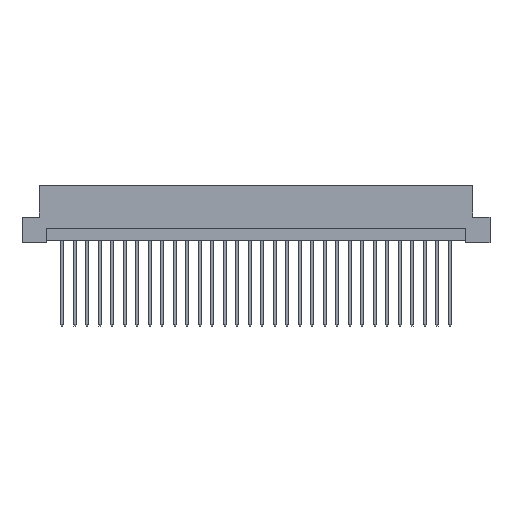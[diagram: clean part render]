
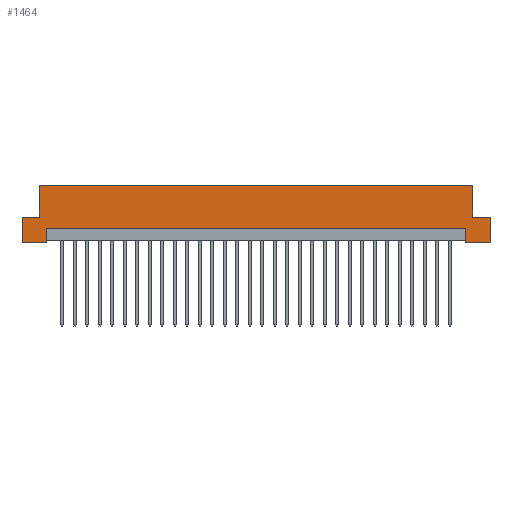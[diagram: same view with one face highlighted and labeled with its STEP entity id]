
A CAD part, front view. The second image highlights one B-rep face of the part: STEP entity #1464.
In plain terms, the highlighted planar face has unit normal (0, -1, 0).
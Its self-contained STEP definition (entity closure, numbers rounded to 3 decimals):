
#237 = EDGE_CURVE ( 'NONE', #8141, #10789, #5623, .T. ) ;
#249 = ORIENTED_EDGE ( 'NONE', *, *, #237, .F. ) ;
#251 = VECTOR ( 'NONE', #8295, 1000. ) ;
#266 = CARTESIAN_POINT ( 'NONE',  ( -44., 0., 5.2 ) ) ;
#455 = EDGE_CURVE ( 'NONE', #5462, #10347, #2420, .T. ) ;
#1003 = DIRECTION ( 'NONE',  ( 0., 0., -1. ) ) ;
#1464 = ADVANCED_FACE ( 'NONE', ( #6351 ), #17099, .F. ) ;
#1670 = VERTEX_POINT ( 'NONE', #11177 ) ;
#1821 = ORIENTED_EDGE ( 'NONE', *, *, #17286, .T. ) ;
#2420 = LINE ( 'NONE', #6477, #3957 ) ;
#2561 = EDGE_CURVE ( 'NONE', #5462, #15795, #7769, .T. ) ;
#2587 = VERTEX_POINT ( 'NONE', #3635 ) ;
#2605 = VECTOR ( 'NONE', #6681, 1000. ) ;
#2892 = CARTESIAN_POINT ( 'NONE',  ( -47.5, 0., 11.6 ) ) ;
#2977 = CARTESIAN_POINT ( 'NONE',  ( -47.5, 0., 5.2 ) ) ;
#3029 = CARTESIAN_POINT ( 'NONE',  ( -47.5, 0., 0. ) ) ;
#3141 = CARTESIAN_POINT ( 'NONE',  ( -47.5, 0., 0. ) ) ;
#3635 = CARTESIAN_POINT ( 'NONE',  ( 44., 0., 5.2 ) ) ;
#3672 = DIRECTION ( 'NONE',  ( 0., 0., -1. ) ) ;
#3743 = DIRECTION ( 'NONE',  ( -1., 0., 0. ) ) ;
#3848 = CARTESIAN_POINT ( 'NONE',  ( 44., 0., 5.2 ) ) ;
#3914 = VECTOR ( 'NONE', #5769, 1000. ) ;
#3940 = EDGE_CURVE ( 'NONE', #1670, #14196, #6947, .T. ) ;
#3957 = VECTOR ( 'NONE', #1003, 1000. ) ;
#4062 = EDGE_CURVE ( 'NONE', #2587, #7244, #14173, .T. ) ;
#4242 = VERTEX_POINT ( 'NONE', #13114 ) ;
#4480 = CARTESIAN_POINT ( 'NONE',  ( 47.5, 0., 5.2 ) ) ;
#4573 = VECTOR ( 'NONE', #10243, 1000. ) ;
#4838 = CARTESIAN_POINT ( 'NONE',  ( 42.6, 0., 2.9 ) ) ;
#5031 = CARTESIAN_POINT ( 'NONE',  ( -47.5, 0., 11.6 ) ) ;
#5462 = VERTEX_POINT ( 'NONE', #4838 ) ;
#5623 = LINE ( 'NONE', #2977, #13481 ) ;
#5658 = CARTESIAN_POINT ( 'NONE',  ( -44., 0., 5.2 ) ) ;
#5728 = CARTESIAN_POINT ( 'NONE',  ( 44., 0., 11.6 ) ) ;
#5769 = DIRECTION ( 'NONE',  ( 0., 0., -1. ) ) ;
#5912 = ORIENTED_EDGE ( 'NONE', *, *, #9536, .F. ) ;
#6019 = VECTOR ( 'NONE', #14844, 1000. ) ;
#6056 = EDGE_LOOP ( 'NONE', ( #10374, #15002, #6068, #13883, #11491, #1821, #12148, #5912, #249, #13480, #8503, #12930 ) ) ;
#6068 = ORIENTED_EDGE ( 'NONE', *, *, #17098, .F. ) ;
#6116 = LINE ( 'NONE', #8852, #3914 ) ;
#6185 = EDGE_CURVE ( 'NONE', #15795, #4242, #7806, .T. ) ;
#6351 = FACE_OUTER_BOUND ( 'NONE', #6056, .T. ) ;
#6477 = CARTESIAN_POINT ( 'NONE',  ( 42.6, 0., 0.5 ) ) ;
#6681 = DIRECTION ( 'NONE',  ( 1., 0., 0. ) ) ;
#6947 = LINE ( 'NONE', #2892, #2605 ) ;
#7089 = DIRECTION ( 'NONE',  ( 0., 0., 1. ) ) ;
#7244 = VERTEX_POINT ( 'NONE', #8250 ) ;
#7387 = DIRECTION ( 'NONE',  ( 1., 0., 0. ) ) ;
#7388 = CARTESIAN_POINT ( 'NONE',  ( -47.5, 0., 5.2 ) ) ;
#7711 = LINE ( 'NONE', #15810, #13461 ) ;
#7769 = LINE ( 'NONE', #10323, #4573 ) ;
#7806 = LINE ( 'NONE', #13180, #13885 ) ;
#8141 = VERTEX_POINT ( 'NONE', #7388 ) ;
#8250 = CARTESIAN_POINT ( 'NONE',  ( 47.5, 0., 5.2 ) ) ;
#8260 = LINE ( 'NONE', #13636, #9953 ) ;
#8295 = DIRECTION ( 'NONE',  ( 0., 0., 1. ) ) ;
#8503 = ORIENTED_EDGE ( 'NONE', *, *, #12013, .F. ) ;
#8852 = CARTESIAN_POINT ( 'NONE',  ( 47.5, 0., 0. ) ) ;
#9001 = CARTESIAN_POINT ( 'NONE',  ( 47.5, 0., 0. ) ) ;
#9334 = DIRECTION ( 'NONE',  ( 0., 1., 0. ) ) ;
#9536 = EDGE_CURVE ( 'NONE', #10789, #1670, #15246, .T. ) ;
#9953 = VECTOR ( 'NONE', #13012, 1000. ) ;
#10243 = DIRECTION ( 'NONE',  ( -1., 0., 0. ) ) ;
#10323 = CARTESIAN_POINT ( 'NONE',  ( 42.6, 0., 2.9 ) ) ;
#10347 = VERTEX_POINT ( 'NONE', #11867 ) ;
#10374 = ORIENTED_EDGE ( 'NONE', *, *, #2561, .F. ) ;
#10403 = DIRECTION ( 'NONE',  ( 0., 0., 1. ) ) ;
#10607 = EDGE_CURVE ( 'NONE', #16990, #8141, #15020, .T. ) ;
#10789 = VERTEX_POINT ( 'NONE', #5658 ) ;
#10998 = AXIS2_PLACEMENT_3D ( 'NONE', #5031, #9334, #10403 ) ;
#11051 = VERTEX_POINT ( 'NONE', #9001 ) ;
#11177 = CARTESIAN_POINT ( 'NONE',  ( -44., 0., 11.6 ) ) ;
#11491 = ORIENTED_EDGE ( 'NONE', *, *, #4062, .F. ) ;
#11867 = CARTESIAN_POINT ( 'NONE',  ( 42.6, 0., 0. ) ) ;
#11900 = EDGE_CURVE ( 'NONE', #7244, #11051, #6116, .T. ) ;
#12013 = EDGE_CURVE ( 'NONE', #4242, #16990, #7711, .T. ) ;
#12148 = ORIENTED_EDGE ( 'NONE', *, *, #3940, .F. ) ;
#12930 = ORIENTED_EDGE ( 'NONE', *, *, #6185, .F. ) ;
#13012 = DIRECTION ( 'NONE',  ( -1., 0., 0. ) ) ;
#13114 = CARTESIAN_POINT ( 'NONE',  ( -42.6, 0., 0. ) ) ;
#13128 = CARTESIAN_POINT ( 'NONE',  ( -42.6, 0., 2.9 ) ) ;
#13180 = CARTESIAN_POINT ( 'NONE',  ( -42.6, 0., 0.5 ) ) ;
#13461 = VECTOR ( 'NONE', #3743, 1000. ) ;
#13480 = ORIENTED_EDGE ( 'NONE', *, *, #10607, .F. ) ;
#13481 = VECTOR ( 'NONE', #14790, 1000. ) ;
#13636 = CARTESIAN_POINT ( 'NONE',  ( -47.5, 0., 0. ) ) ;
#13787 = VECTOR ( 'NONE', #7089, 1000. ) ;
#13883 = ORIENTED_EDGE ( 'NONE', *, *, #11900, .F. ) ;
#13885 = VECTOR ( 'NONE', #3672, 1000. ) ;
#14173 = LINE ( 'NONE', #4480, #15853 ) ;
#14196 = VERTEX_POINT ( 'NONE', #5728 ) ;
#14790 = DIRECTION ( 'NONE',  ( 1., 0., 0. ) ) ;
#14844 = DIRECTION ( 'NONE',  ( 0., 0., 1. ) ) ;
#15002 = ORIENTED_EDGE ( 'NONE', *, *, #455, .T. ) ;
#15020 = LINE ( 'NONE', #3029, #13787 ) ;
#15246 = LINE ( 'NONE', #266, #251 ) ;
#15795 = VERTEX_POINT ( 'NONE', #13128 ) ;
#15810 = CARTESIAN_POINT ( 'NONE',  ( -47.5, 0., 0. ) ) ;
#15853 = VECTOR ( 'NONE', #7387, 1000. ) ;
#16990 = VERTEX_POINT ( 'NONE', #3141 ) ;
#17098 = EDGE_CURVE ( 'NONE', #11051, #10347, #8260, .T. ) ;
#17099 = PLANE ( 'NONE',  #10998 ) ;
#17286 = EDGE_CURVE ( 'NONE', #2587, #14196, #17321, .T. ) ;
#17321 = LINE ( 'NONE', #3848, #6019 ) ;
